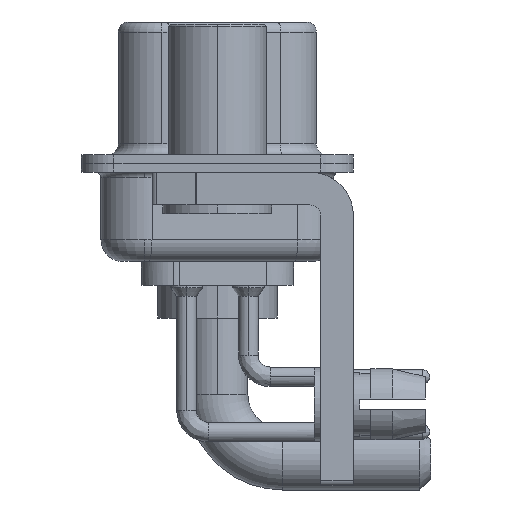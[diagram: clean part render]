
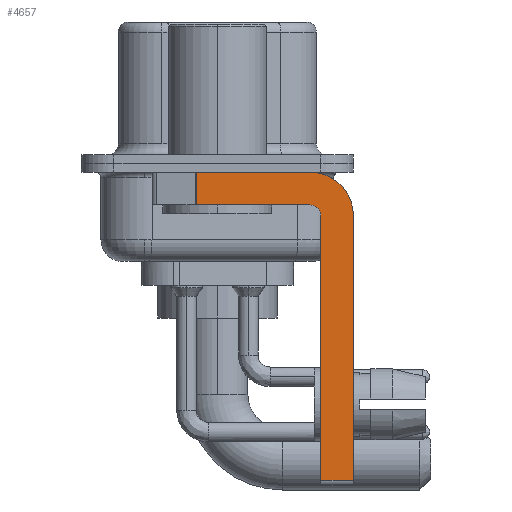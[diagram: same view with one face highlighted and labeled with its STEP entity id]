
A CAD part, left-side view. The second image highlights one B-rep face of the part: STEP entity #4657.
In plain terms, the highlighted planar face has unit normal (-1, 0, 0).
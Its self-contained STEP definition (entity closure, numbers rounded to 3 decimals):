
#536 = CARTESIAN_POINT ( 'NONE',  ( -2.9, -4.25, -1.9 ) ) ;
#1161 = LINE ( 'NONE', #17411, #21447 ) ;
#2209 = AXIS2_PLACEMENT_3D ( 'NONE', #9728, #23831, #11574 ) ;
#2716 = ORIENTED_EDGE ( 'NONE', *, *, #8231, .F. ) ;
#3924 = VECTOR ( 'NONE', #15686, 1000. ) ;
#4170 = VERTEX_POINT ( 'NONE', #6546 ) ;
#4657 = ADVANCED_FACE ( 'NONE', ( #8648 ), #6509, .F. ) ;
#4790 = VERTEX_POINT ( 'NONE', #7409 ) ;
#5097 = CARTESIAN_POINT ( 'NONE',  ( -2.9, -4.25, -14.55 ) ) ;
#5161 = VECTOR ( 'NONE', #24944, 1000. ) ;
#5196 = VERTEX_POINT ( 'NONE', #25635 ) ;
#5430 = CARTESIAN_POINT ( 'NONE',  ( -2.9, -6.25, -2.4 ) ) ;
#5544 = DIRECTION ( 'NONE',  ( 0., -1., 0. ) ) ;
#6357 = DIRECTION ( 'NONE',  ( 1., 0., 0. ) ) ;
#6509 = PLANE ( 'NONE',  #28184 ) ;
#6546 = CARTESIAN_POINT ( 'NONE',  ( -2.9, -4.75, -2.4 ) ) ;
#7286 = EDGE_CURVE ( 'NONE', #19599, #4790, #18775, .T. ) ;
#7409 = CARTESIAN_POINT ( 'NONE',  ( -2.9, -6.25, -14.55 ) ) ;
#7981 = CARTESIAN_POINT ( 'NONE',  ( -2.9, -6.25, -2.4 ) ) ;
#8231 = EDGE_CURVE ( 'NONE', #4170, #14700, #25967, .T. ) ;
#8647 = ORIENTED_EDGE ( 'NONE', *, *, #20599, .F. ) ;
#8648 = FACE_OUTER_BOUND ( 'NONE', #15271, .T. ) ;
#9298 = EDGE_CURVE ( 'NONE', #17326, #23397, #28685, .T. ) ;
#9675 = DIRECTION ( 'NONE',  ( 1., 0., 0. ) ) ;
#9728 = CARTESIAN_POINT ( 'NONE',  ( -2.9, -4.25, -2.4 ) ) ;
#9797 = DIRECTION ( 'NONE',  ( 0., 1., 0. ) ) ;
#9903 = ORIENTED_EDGE ( 'NONE', *, *, #11193, .F. ) ;
#10096 = LINE ( 'NONE', #536, #18256 ) ;
#10391 = LINE ( 'NONE', #26641, #5161 ) ;
#10539 = LINE ( 'NONE', #12966, #3924 ) ;
#11064 = DIRECTION ( 'NONE',  ( 0., 0., -1. ) ) ;
#11193 = EDGE_CURVE ( 'NONE', #23397, #4790, #28769, .T. ) ;
#11574 = DIRECTION ( 'NONE',  ( 0., 0., 1. ) ) ;
#11736 = ORIENTED_EDGE ( 'NONE', *, *, #13462, .F. ) ;
#12229 = EDGE_CURVE ( 'NONE', #5196, #17326, #10539, .T. ) ;
#12593 = VECTOR ( 'NONE', #17519, 1000. ) ;
#12861 = DIRECTION ( 'NONE',  ( 0., 0., 1. ) ) ;
#12966 = CARTESIAN_POINT ( 'NONE',  ( -2.9, 3., -0.4 ) ) ;
#13462 = EDGE_CURVE ( 'NONE', #19599, #4170, #1161, .T. ) ;
#14700 = VERTEX_POINT ( 'NONE', #29100 ) ;
#15271 = EDGE_LOOP ( 'NONE', ( #20719, #18340, #8647, #2716, #11736, #15345, #9903, #26724 ) ) ;
#15345 = ORIENTED_EDGE ( 'NONE', *, *, #7286, .T. ) ;
#15598 = AXIS2_PLACEMENT_3D ( 'NONE', #16355, #9675, #28198 ) ;
#15686 = DIRECTION ( 'NONE',  ( 0., -1., 0. ) ) ;
#16355 = CARTESIAN_POINT ( 'NONE',  ( -2.9, -4.25, -2.4 ) ) ;
#17202 = VECTOR ( 'NONE', #5544, 1000. ) ;
#17326 = VERTEX_POINT ( 'NONE', #25007 ) ;
#17411 = CARTESIAN_POINT ( 'NONE',  ( -2.9, -4.75, -14.8 ) ) ;
#17519 = DIRECTION ( 'NONE',  ( 0., 0., -1. ) ) ;
#18256 = VECTOR ( 'NONE', #9797, 1000. ) ;
#18340 = ORIENTED_EDGE ( 'NONE', *, *, #19133, .T. ) ;
#18775 = LINE ( 'NONE', #5097, #17202 ) ;
#19133 = EDGE_CURVE ( 'NONE', #5196, #19441, #10391, .T. ) ;
#19441 = VERTEX_POINT ( 'NONE', #23856 ) ;
#19599 = VERTEX_POINT ( 'NONE', #22478 ) ;
#20599 = EDGE_CURVE ( 'NONE', #14700, #19441, #10096, .T. ) ;
#20719 = ORIENTED_EDGE ( 'NONE', *, *, #12229, .F. ) ;
#21447 = VECTOR ( 'NONE', #12861, 1000. ) ;
#22478 = CARTESIAN_POINT ( 'NONE',  ( -2.9, -4.75, -14.55 ) ) ;
#23397 = VERTEX_POINT ( 'NONE', #5430 ) ;
#23831 = DIRECTION ( 'NONE',  ( -1., 0., 0. ) ) ;
#23856 = CARTESIAN_POINT ( 'NONE',  ( -2.9, 0.978, -1.9 ) ) ;
#24944 = DIRECTION ( 'NONE',  ( 0., 0., -1. ) ) ;
#25007 = CARTESIAN_POINT ( 'NONE',  ( -2.9, -4.25, -0.4 ) ) ;
#25635 = CARTESIAN_POINT ( 'NONE',  ( -2.9, 0.978, -0.4 ) ) ;
#25967 = CIRCLE ( 'NONE', #2209, 0.5 ) ;
#26641 = CARTESIAN_POINT ( 'NONE',  ( -2.9, 0.978, -1.9 ) ) ;
#26724 = ORIENTED_EDGE ( 'NONE', *, *, #9298, .F. ) ;
#27158 = CARTESIAN_POINT ( 'NONE',  ( -2.9, -4.25, -2.4 ) ) ;
#28184 = AXIS2_PLACEMENT_3D ( 'NONE', #27158, #6357, #11064 ) ;
#28198 = DIRECTION ( 'NONE',  ( 0., 0., -1. ) ) ;
#28685 = CIRCLE ( 'NONE', #15598, 2. ) ;
#28769 = LINE ( 'NONE', #7981, #12593 ) ;
#29100 = CARTESIAN_POINT ( 'NONE',  ( -2.9, -4.25, -1.9 ) ) ;
